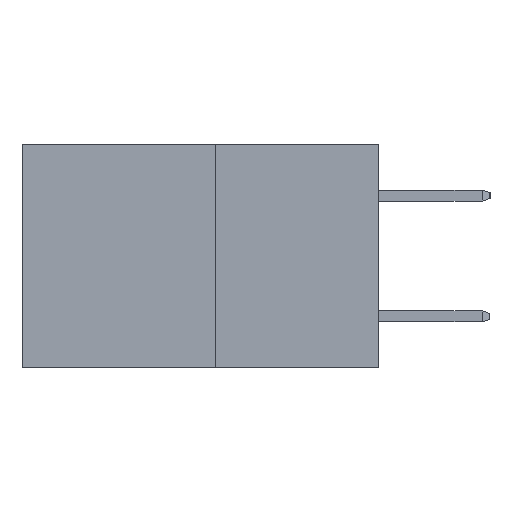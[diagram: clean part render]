
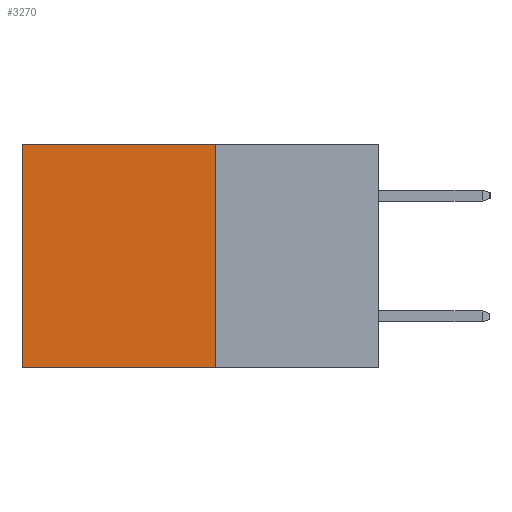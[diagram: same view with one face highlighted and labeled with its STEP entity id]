
A CAD part, left-side view. The second image highlights one B-rep face of the part: STEP entity #3270.
In plain terms, the highlighted planar face has unit normal (-1, 0, 0).
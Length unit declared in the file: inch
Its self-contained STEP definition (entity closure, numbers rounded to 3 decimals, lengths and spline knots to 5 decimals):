
#286 = CARTESIAN_POINT ( 'NONE',  ( 0.277, 0.59, -0.37 ) ) ;
#506 = FACE_OUTER_BOUND ( 'NONE', #2056, .T. ) ;
#532 = DIRECTION ( 'NONE',  ( 1., 0., 0. ) ) ;
#589 = PLANE ( 'NONE',  #8052 ) ;
#1155 = ORIENTED_EDGE ( 'NONE', *, *, #6323, .F. ) ;
#1483 = CARTESIAN_POINT ( 'NONE',  ( 0.277, 0.27, -0.37 ) ) ;
#1605 = DIRECTION ( 'NONE',  ( 0., 0., -1. ) ) ;
#1656 = VECTOR ( 'NONE', #6139, 39.37008 ) ;
#2056 = EDGE_LOOP ( 'NONE', ( #6662, #1155, #3247, #3490 ) ) ;
#2671 = CARTESIAN_POINT ( 'NONE',  ( 0.277, 0.27, -0.37 ) ) ;
#2798 = LINE ( 'NONE', #8542, #6470 ) ;
#2805 = VERTEX_POINT ( 'NONE', #6253 ) ;
#2919 = DIRECTION ( 'NONE',  ( 0., 0., -1. ) ) ;
#2972 = CARTESIAN_POINT ( 'NONE',  ( 0.277, 0.59, -0.37 ) ) ;
#3183 = LINE ( 'NONE', #4792, #8676 ) ;
#3247 = ORIENTED_EDGE ( 'NONE', *, *, #5949, .F. ) ;
#3270 = ADVANCED_FACE ( 'NONE', ( #506 ), #589, .F. ) ;
#3490 = ORIENTED_EDGE ( 'NONE', *, *, #9137, .T. ) ;
#4792 = CARTESIAN_POINT ( 'NONE',  ( 0.277, 0.27, 0. ) ) ;
#5412 = LINE ( 'NONE', #2972, #8961 ) ;
#5781 = VERTEX_POINT ( 'NONE', #286 ) ;
#5949 = EDGE_CURVE ( 'NONE', #7030, #8931, #2798, .T. ) ;
#5953 = CARTESIAN_POINT ( 'NONE',  ( 0.277, 0.27, -0.37 ) ) ;
#6139 = DIRECTION ( 'NONE',  ( 0., 1., 0. ) ) ;
#6253 = CARTESIAN_POINT ( 'NONE',  ( 0.277, 0.59, 0. ) ) ;
#6323 = EDGE_CURVE ( 'NONE', #8931, #5781, #9410, .T. ) ;
#6470 = VECTOR ( 'NONE', #8437, 39.37008 ) ;
#6662 = ORIENTED_EDGE ( 'NONE', *, *, #8357, .T. ) ;
#6912 = CARTESIAN_POINT ( 'NONE',  ( 0.277, 0.27, 0. ) ) ;
#7030 = VERTEX_POINT ( 'NONE', #6912 ) ;
#8052 = AXIS2_PLACEMENT_3D ( 'NONE', #2671, #532, #1605 ) ;
#8329 = DIRECTION ( 'NONE',  ( 0., 1., 0. ) ) ;
#8357 = EDGE_CURVE ( 'NONE', #2805, #5781, #5412, .T. ) ;
#8437 = DIRECTION ( 'NONE',  ( 0., 0., -1. ) ) ;
#8542 = CARTESIAN_POINT ( 'NONE',  ( 0.277, 0.27, -0.37 ) ) ;
#8676 = VECTOR ( 'NONE', #8329, 39.37008 ) ;
#8931 = VERTEX_POINT ( 'NONE', #1483 ) ;
#8961 = VECTOR ( 'NONE', #2919, 39.37008 ) ;
#9137 = EDGE_CURVE ( 'NONE', #7030, #2805, #3183, .T. ) ;
#9410 = LINE ( 'NONE', #5953, #1656 ) ;
